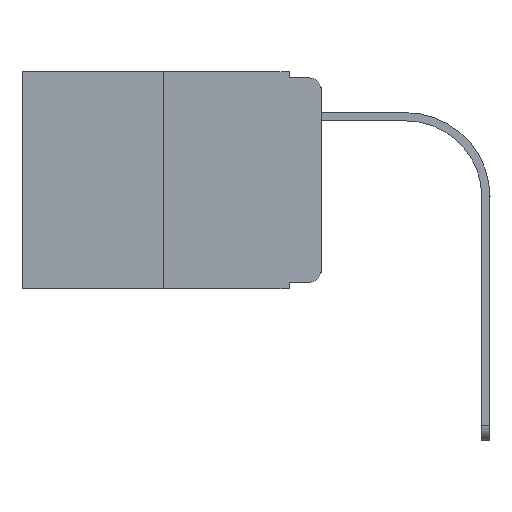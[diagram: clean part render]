
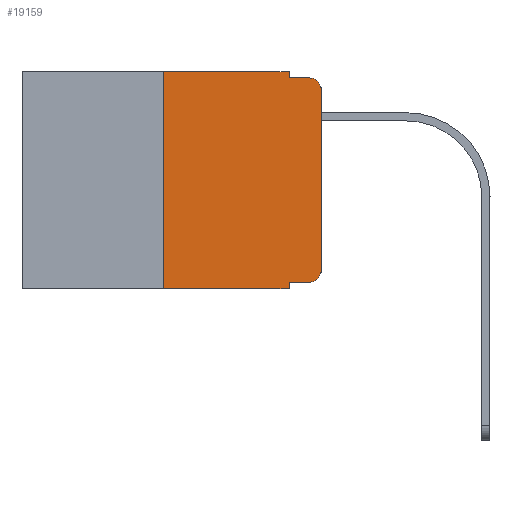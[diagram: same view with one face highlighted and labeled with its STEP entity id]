
A CAD part, left-side view. The second image highlights one B-rep face of the part: STEP entity #19159.
In plain terms, the highlighted planar face has unit normal (-1, 0, 0).
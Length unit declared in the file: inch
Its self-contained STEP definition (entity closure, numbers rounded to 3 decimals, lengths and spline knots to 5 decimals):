
#56 = CARTESIAN_POINT ( 'NONE',  ( 0., 0.02, -0.03 ) ) ;
#274 = EDGE_CURVE ( 'NONE', #17591, #2811, #7023, .T. ) ;
#378 = CARTESIAN_POINT ( 'NONE',  ( 0., 0.25, 0. ) ) ;
#399 = CARTESIAN_POINT ( 'NONE',  ( 0., 0.02, -0.333 ) ) ;
#688 = CARTESIAN_POINT ( 'NONE',  ( 0., 0.473, 0. ) ) ;
#820 = ORIENTED_EDGE ( 'NONE', *, *, #14229, .T. ) ;
#966 = EDGE_CURVE ( 'NONE', #10584, #12064, #15737, .T. ) ;
#1123 = ORIENTED_EDGE ( 'NONE', *, *, #11850, .T. ) ;
#1140 = ORIENTED_EDGE ( 'NONE', *, *, #274, .T. ) ;
#1255 = VECTOR ( 'NONE', #1737, 39.37008 ) ;
#1737 = DIRECTION ( 'NONE',  ( 0., -1., 0. ) ) ;
#1839 = EDGE_CURVE ( 'NONE', #8987, #11382, #12866, .T. ) ;
#2387 = VECTOR ( 'NONE', #18128, 39.37008 ) ;
#2811 = VERTEX_POINT ( 'NONE', #17045 ) ;
#3451 = CARTESIAN_POINT ( 'NONE',  ( 0., 0.051, -0.01 ) ) ;
#3764 = LINE ( 'NONE', #10035, #2387 ) ;
#3800 = VECTOR ( 'NONE', #6381, 39.37008 ) ;
#4353 = ORIENTED_EDGE ( 'NONE', *, *, #11723, .T. ) ;
#4372 = DIRECTION ( 'NONE',  ( -1., 0., 0. ) ) ;
#4459 = EDGE_CURVE ( 'NONE', #2811, #18987, #3764, .T. ) ;
#4479 = DIRECTION ( 'NONE',  ( 0., 0., -1. ) ) ;
#4690 = ORIENTED_EDGE ( 'NONE', *, *, #8214, .F. ) ;
#4740 = DIRECTION ( 'NONE',  ( 1., 0., 0. ) ) ;
#4859 = ORIENTED_EDGE ( 'NONE', *, *, #966, .F. ) ;
#5000 = CARTESIAN_POINT ( 'NONE',  ( 0., 0.02, -0.01 ) ) ;
#5297 = CARTESIAN_POINT ( 'NONE',  ( 0., 0.473, -0.343 ) ) ;
#5699 = CARTESIAN_POINT ( 'NONE',  ( 0., 0.051, -0.333 ) ) ;
#6004 = VERTEX_POINT ( 'NONE', #3451 ) ;
#6277 = PLANE ( 'NONE',  #12413 ) ;
#6381 = DIRECTION ( 'NONE',  ( 0., 0., -1. ) ) ;
#6414 = VERTEX_POINT ( 'NONE', #13450 ) ;
#6753 = LINE ( 'NONE', #11224, #8459 ) ;
#6959 = DIRECTION ( 'NONE',  ( 0., -1., 0. ) ) ;
#7023 = CIRCLE ( 'NONE', #12331, 0.02 ) ;
#7341 = CARTESIAN_POINT ( 'NONE',  ( 0., 0.02, -0.313 ) ) ;
#7803 = VECTOR ( 'NONE', #6959, 39.37008 ) ;
#8214 = EDGE_CURVE ( 'NONE', #6414, #6004, #12500, .T. ) ;
#8459 = VECTOR ( 'NONE', #19410, 39.37008 ) ;
#8813 = CARTESIAN_POINT ( 'NONE',  ( 0., 0.25, -0.343 ) ) ;
#8987 = VERTEX_POINT ( 'NONE', #8813 ) ;
#9468 = VECTOR ( 'NONE', #19185, 39.37008 ) ;
#9784 = DIRECTION ( 'NONE',  ( 0., 0., -1. ) ) ;
#10035 = CARTESIAN_POINT ( 'NONE',  ( 0., 0., 0. ) ) ;
#10145 = EDGE_CURVE ( 'NONE', #6004, #13984, #6753, .T. ) ;
#10584 = VERTEX_POINT ( 'NONE', #18971 ) ;
#10698 = ORIENTED_EDGE ( 'NONE', *, *, #10145, .F. ) ;
#10727 = ORIENTED_EDGE ( 'NONE', *, *, #19332, .F. ) ;
#11224 = CARTESIAN_POINT ( 'NONE',  ( 0., 0.051, -0.01 ) ) ;
#11248 = DIRECTION ( 'NONE',  ( 0., 0., -1. ) ) ;
#11354 = EDGE_LOOP ( 'NONE', ( #15585, #4353, #10698, #4690, #10727, #16142, #1123, #4859, #820, #1140 ) ) ;
#11382 = VERTEX_POINT ( 'NONE', #378 ) ;
#11421 = CIRCLE ( 'NONE', #14107, 0.02 ) ;
#11723 = EDGE_CURVE ( 'NONE', #18987, #13984, #11421, .T. ) ;
#11850 = EDGE_CURVE ( 'NONE', #8987, #12064, #19089, .T. ) ;
#11909 = LINE ( 'NONE', #5699, #12847 ) ;
#12064 = VERTEX_POINT ( 'NONE', #13896 ) ;
#12242 = DIRECTION ( 'NONE',  ( -1., 0., 0. ) ) ;
#12331 = AXIS2_PLACEMENT_3D ( 'NONE', #7341, #4372, #4479 ) ;
#12372 = CARTESIAN_POINT ( 'NONE',  ( 0., 0., -0.03 ) ) ;
#12413 = AXIS2_PLACEMENT_3D ( 'NONE', #16107, #4740, #9784 ) ;
#12500 = LINE ( 'NONE', #17390, #3800 ) ;
#12847 = VECTOR ( 'NONE', #18240, 39.37008 ) ;
#12866 = LINE ( 'NONE', #19493, #9468 ) ;
#13450 = CARTESIAN_POINT ( 'NONE',  ( 0., 0.051, 0. ) ) ;
#13896 = CARTESIAN_POINT ( 'NONE',  ( 0., 0.051, -0.343 ) ) ;
#13984 = VERTEX_POINT ( 'NONE', #5000 ) ;
#14107 = AXIS2_PLACEMENT_3D ( 'NONE', #56, #12242, #18786 ) ;
#14229 = EDGE_CURVE ( 'NONE', #10584, #17591, #11909, .T. ) ;
#14865 = LINE ( 'NONE', #688, #7803 ) ;
#15585 = ORIENTED_EDGE ( 'NONE', *, *, #4459, .T. ) ;
#15737 = LINE ( 'NONE', #19139, #16043 ) ;
#16043 = VECTOR ( 'NONE', #11248, 39.37008 ) ;
#16107 = CARTESIAN_POINT ( 'NONE',  ( 0., 0.473, 0. ) ) ;
#16142 = ORIENTED_EDGE ( 'NONE', *, *, #1839, .F. ) ;
#17045 = CARTESIAN_POINT ( 'NONE',  ( 0., 0., -0.313 ) ) ;
#17390 = CARTESIAN_POINT ( 'NONE',  ( 0., 0.051, 0. ) ) ;
#17591 = VERTEX_POINT ( 'NONE', #399 ) ;
#18128 = DIRECTION ( 'NONE',  ( 0., 0., 1. ) ) ;
#18240 = DIRECTION ( 'NONE',  ( 0., -1., 0. ) ) ;
#18786 = DIRECTION ( 'NONE',  ( 0., 0., -1. ) ) ;
#18904 = FACE_OUTER_BOUND ( 'NONE', #11354, .T. ) ;
#18971 = CARTESIAN_POINT ( 'NONE',  ( 0., 0.051, -0.333 ) ) ;
#18987 = VERTEX_POINT ( 'NONE', #12372 ) ;
#19089 = LINE ( 'NONE', #5297, #1255 ) ;
#19139 = CARTESIAN_POINT ( 'NONE',  ( 0., 0.051, 0. ) ) ;
#19159 = ADVANCED_FACE ( 'NONE', ( #18904 ), #6277, .F. ) ;
#19185 = DIRECTION ( 'NONE',  ( 0., 0., 1. ) ) ;
#19332 = EDGE_CURVE ( 'NONE', #11382, #6414, #14865, .T. ) ;
#19410 = DIRECTION ( 'NONE',  ( 0., -1., 0. ) ) ;
#19493 = CARTESIAN_POINT ( 'NONE',  ( 0., 0.25, 0. ) ) ;
